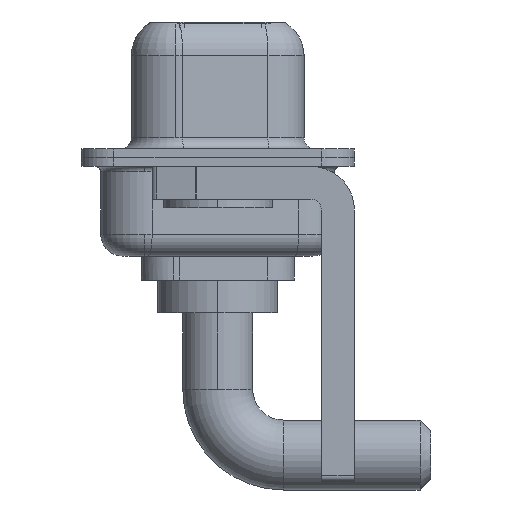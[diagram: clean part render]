
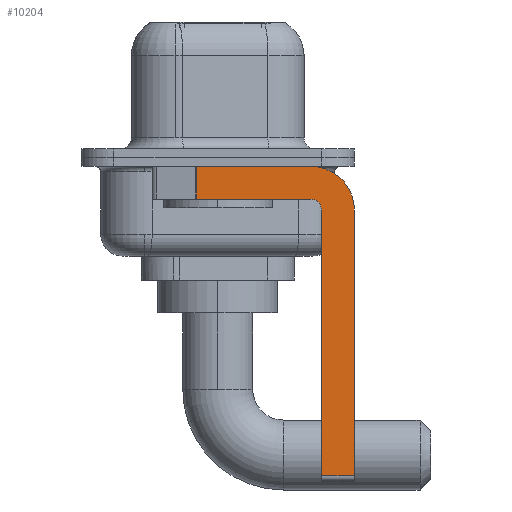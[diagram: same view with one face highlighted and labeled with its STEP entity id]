
A CAD part, left-side view. The second image highlights one B-rep face of the part: STEP entity #10204.
In plain terms, the highlighted planar face has unit normal (-1, 0, 0).
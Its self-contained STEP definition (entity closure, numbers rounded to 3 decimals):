
#255 = CARTESIAN_POINT ( 'NONE',  ( -2.9, -4.75, -2.4 ) ) ;
#372 = EDGE_CURVE ( 'NONE', #13281, #7535, #8124, .T. ) ;
#775 = DIRECTION ( 'NONE',  ( 0., -1., 0. ) ) ;
#967 = LINE ( 'NONE', #9650, #10888 ) ;
#982 = LINE ( 'NONE', #5345, #9733 ) ;
#1095 = VECTOR ( 'NONE', #9528, 1000. ) ;
#1346 = ORIENTED_EDGE ( 'NONE', *, *, #9782, .T. ) ;
#1485 = VERTEX_POINT ( 'NONE', #13183 ) ;
#1683 = DIRECTION ( 'NONE',  ( 0., 0., -1. ) ) ;
#1912 = CARTESIAN_POINT ( 'NONE',  ( -2.9, -4.25, -14.55 ) ) ;
#2045 = ORIENTED_EDGE ( 'NONE', *, *, #372, .F. ) ;
#2086 = CARTESIAN_POINT ( 'NONE',  ( -2.9, 0.978, -1.9 ) ) ;
#2471 = LINE ( 'NONE', #5673, #9392 ) ;
#2554 = CARTESIAN_POINT ( 'NONE',  ( -2.9, -4.25, -2.4 ) ) ;
#2750 = EDGE_LOOP ( 'NONE', ( #2045, #12428, #9005, #5231, #5899, #1346, #3220, #7742 ) ) ;
#3220 = ORIENTED_EDGE ( 'NONE', *, *, #6322, .F. ) ;
#3400 = CARTESIAN_POINT ( 'NONE',  ( -2.9, -6.25, -14.55 ) ) ;
#3535 = PLANE ( 'NONE',  #6323 ) ;
#3833 = CARTESIAN_POINT ( 'NONE',  ( -2.9, -4.25, -1.9 ) ) ;
#4533 = CARTESIAN_POINT ( 'NONE',  ( -2.9, -4.25, -2.4 ) ) ;
#4629 = EDGE_CURVE ( 'NONE', #7535, #1485, #7876, .T. ) ;
#4767 = CARTESIAN_POINT ( 'NONE',  ( -2.9, -4.75, -14.55 ) ) ;
#4942 = VECTOR ( 'NONE', #775, 1000. ) ;
#5231 = ORIENTED_EDGE ( 'NONE', *, *, #8551, .F. ) ;
#5345 = CARTESIAN_POINT ( 'NONE',  ( -2.9, -4.75, -14.8 ) ) ;
#5673 = CARTESIAN_POINT ( 'NONE',  ( -2.9, -6.25, -2.4 ) ) ;
#5858 = VERTEX_POINT ( 'NONE', #4767 ) ;
#5899 = ORIENTED_EDGE ( 'NONE', *, *, #11115, .F. ) ;
#6065 = CARTESIAN_POINT ( 'NONE',  ( -2.9, 3., -0.4 ) ) ;
#6322 = EDGE_CURVE ( 'NONE', #1485, #12440, #2471, .T. ) ;
#6323 = AXIS2_PLACEMENT_3D ( 'NONE', #2554, #12364, #1683 ) ;
#6749 = DIRECTION ( 'NONE',  ( 0., 0., -1. ) ) ;
#7275 = DIRECTION ( 'NONE',  ( 0., 0., 1. ) ) ;
#7535 = VERTEX_POINT ( 'NONE', #10715 ) ;
#7646 = LINE ( 'NONE', #12033, #11551 ) ;
#7685 = CARTESIAN_POINT ( 'NONE',  ( -2.9, -4.25, -2.4 ) ) ;
#7742 = ORIENTED_EDGE ( 'NONE', *, *, #4629, .F. ) ;
#7830 = DIRECTION ( 'NONE',  ( 1., 0., 0. ) ) ;
#7876 = CIRCLE ( 'NONE', #12863, 2. ) ;
#7972 = FACE_OUTER_BOUND ( 'NONE', #2750, .T. ) ;
#8124 = LINE ( 'NONE', #6065, #4942 ) ;
#8233 = VERTEX_POINT ( 'NONE', #2086 ) ;
#8551 = EDGE_CURVE ( 'NONE', #11752, #11557, #11303, .T. ) ;
#9005 = ORIENTED_EDGE ( 'NONE', *, *, #11701, .F. ) ;
#9392 = VECTOR ( 'NONE', #10005, 1000. ) ;
#9528 = DIRECTION ( 'NONE',  ( 0., -1., 0. ) ) ;
#9650 = CARTESIAN_POINT ( 'NONE',  ( -2.9, -4.25, -1.9 ) ) ;
#9733 = VECTOR ( 'NONE', #7275, 1000. ) ;
#9735 = LINE ( 'NONE', #1912, #1095 ) ;
#9782 = EDGE_CURVE ( 'NONE', #5858, #12440, #9735, .T. ) ;
#9968 = DIRECTION ( 'NONE',  ( 0., 0., -1. ) ) ;
#10005 = DIRECTION ( 'NONE',  ( 0., 0., -1. ) ) ;
#10204 = ADVANCED_FACE ( 'NONE', ( #7972 ), #3535, .F. ) ;
#10299 = DIRECTION ( 'NONE',  ( -1., 0., 0. ) ) ;
#10715 = CARTESIAN_POINT ( 'NONE',  ( -2.9, -4.25, -0.4 ) ) ;
#10862 = EDGE_CURVE ( 'NONE', #13281, #8233, #7646, .T. ) ;
#10888 = VECTOR ( 'NONE', #11510, 1000. ) ;
#11115 = EDGE_CURVE ( 'NONE', #5858, #11752, #982, .T. ) ;
#11303 = CIRCLE ( 'NONE', #11982, 0.5 ) ;
#11510 = DIRECTION ( 'NONE',  ( 0., 1., 0. ) ) ;
#11551 = VECTOR ( 'NONE', #9968, 1000. ) ;
#11557 = VERTEX_POINT ( 'NONE', #3833 ) ;
#11701 = EDGE_CURVE ( 'NONE', #11557, #8233, #967, .T. ) ;
#11752 = VERTEX_POINT ( 'NONE', #255 ) ;
#11982 = AXIS2_PLACEMENT_3D ( 'NONE', #7685, #10299, #12011 ) ;
#12011 = DIRECTION ( 'NONE',  ( 0., 0., 1. ) ) ;
#12033 = CARTESIAN_POINT ( 'NONE',  ( -2.9, 0.978, -1.9 ) ) ;
#12364 = DIRECTION ( 'NONE',  ( 1., 0., 0. ) ) ;
#12428 = ORIENTED_EDGE ( 'NONE', *, *, #10862, .T. ) ;
#12440 = VERTEX_POINT ( 'NONE', #3400 ) ;
#12863 = AXIS2_PLACEMENT_3D ( 'NONE', #4533, #7830, #6749 ) ;
#13183 = CARTESIAN_POINT ( 'NONE',  ( -2.9, -6.25, -2.4 ) ) ;
#13281 = VERTEX_POINT ( 'NONE', #13327 ) ;
#13327 = CARTESIAN_POINT ( 'NONE',  ( -2.9, 0.978, -0.4 ) ) ;
